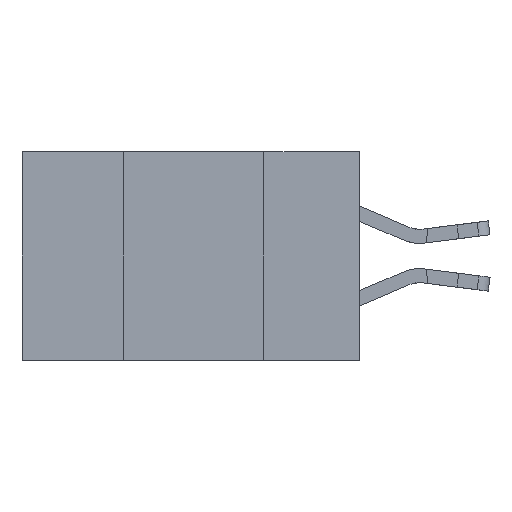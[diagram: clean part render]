
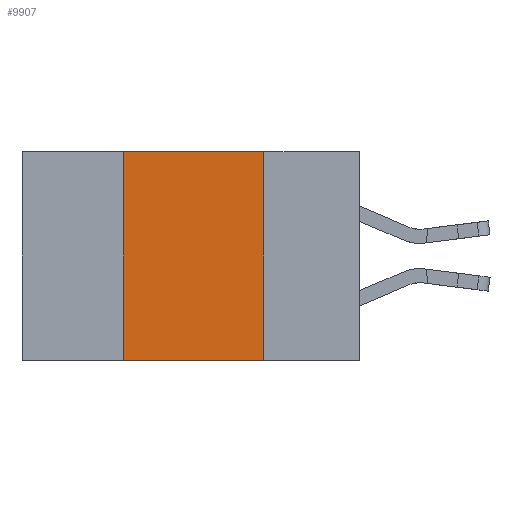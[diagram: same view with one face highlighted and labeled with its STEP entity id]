
A CAD part, left-side view. The second image highlights one B-rep face of the part: STEP entity #9907.
In plain terms, the highlighted planar face has unit normal (-1, 0, 0).
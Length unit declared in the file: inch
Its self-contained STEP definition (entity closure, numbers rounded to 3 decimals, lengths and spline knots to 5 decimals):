
#1948 = ORIENTED_EDGE ( 'NONE', *, *, #9375, .T. ) ;
#3151 = VECTOR ( 'NONE', #23013, 39.37008 ) ;
#3332 = ORIENTED_EDGE ( 'NONE', *, *, #14054, .F. ) ;
#4099 = LINE ( 'NONE', #23434, #21672 ) ;
#5461 = CARTESIAN_POINT ( 'NONE',  ( 0., 0.6, 0. ) ) ;
#6043 = CARTESIAN_POINT ( 'NONE',  ( 0., 0.17, -0.37 ) ) ;
#9229 = DIRECTION ( 'NONE',  ( 0., 0., -1. ) ) ;
#9315 = PLANE ( 'NONE',  #21964 ) ;
#9375 = EDGE_CURVE ( 'NONE', #21737, #24092, #15410, .T. ) ;
#9864 = VECTOR ( 'NONE', #22477, 39.37008 ) ;
#9907 = ADVANCED_FACE ( 'NONE', ( #12269 ), #9315, .F. ) ;
#10360 = EDGE_CURVE ( 'NONE', #13770, #21700, #17865, .T. ) ;
#12269 = FACE_OUTER_BOUND ( 'NONE', #16453, .T. ) ;
#12355 = ORIENTED_EDGE ( 'NONE', *, *, #24037, .F. ) ;
#12578 = CARTESIAN_POINT ( 'NONE',  ( 0., 0.42, 0. ) ) ;
#13770 = VERTEX_POINT ( 'NONE', #12578 ) ;
#14054 = EDGE_CURVE ( 'NONE', #21700, #24092, #24098, .T. ) ;
#15311 = CARTESIAN_POINT ( 'NONE',  ( 0., 0.42, -0.37 ) ) ;
#15410 = LINE ( 'NONE', #18537, #9864 ) ;
#16453 = EDGE_LOOP ( 'NONE', ( #3332, #18278, #12355, #1948 ) ) ;
#16554 = DIRECTION ( 'NONE',  ( 0., -1., 0. ) ) ;
#17865 = LINE ( 'NONE', #20337, #22444 ) ;
#18278 = ORIENTED_EDGE ( 'NONE', *, *, #10360, .F. ) ;
#18537 = CARTESIAN_POINT ( 'NONE',  ( 0., 0.6, -0.37 ) ) ;
#19038 = CARTESIAN_POINT ( 'NONE',  ( 0., 0.17, 0. ) ) ;
#20337 = CARTESIAN_POINT ( 'NONE',  ( 0., 0.6, 0. ) ) ;
#21672 = VECTOR ( 'NONE', #23529, 39.37008 ) ;
#21700 = VERTEX_POINT ( 'NONE', #19038 ) ;
#21737 = VERTEX_POINT ( 'NONE', #15311 ) ;
#21964 = AXIS2_PLACEMENT_3D ( 'NONE', #5461, #23185, #9229 ) ;
#22444 = VECTOR ( 'NONE', #16554, 39.37008 ) ;
#22477 = DIRECTION ( 'NONE',  ( 0., -1., 0. ) ) ;
#23013 = DIRECTION ( 'NONE',  ( 0., 0., -1. ) ) ;
#23185 = DIRECTION ( 'NONE',  ( 1., 0., 0. ) ) ;
#23365 = CARTESIAN_POINT ( 'NONE',  ( 0., 0.17, 0. ) ) ;
#23434 = CARTESIAN_POINT ( 'NONE',  ( 0., 0.42, 0. ) ) ;
#23529 = DIRECTION ( 'NONE',  ( 0., 0., 1. ) ) ;
#24037 = EDGE_CURVE ( 'NONE', #21737, #13770, #4099, .T. ) ;
#24092 = VERTEX_POINT ( 'NONE', #6043 ) ;
#24098 = LINE ( 'NONE', #23365, #3151 ) ;
